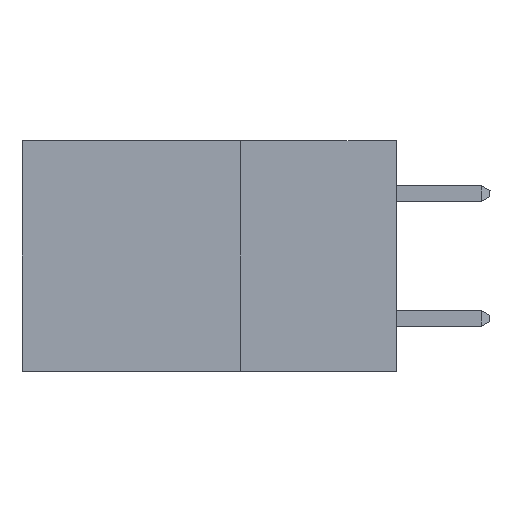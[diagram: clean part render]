
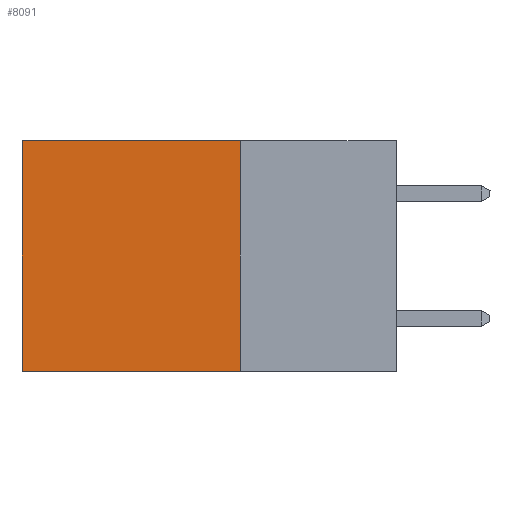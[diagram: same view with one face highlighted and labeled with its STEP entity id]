
A CAD part, left-side view. The second image highlights one B-rep face of the part: STEP entity #8091.
In plain terms, the highlighted planar face has unit normal (-1, 0, 0).
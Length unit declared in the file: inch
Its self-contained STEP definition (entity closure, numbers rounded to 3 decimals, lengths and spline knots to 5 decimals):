
#613 = CARTESIAN_POINT ( 'NONE',  ( 0.298, 0.6, 0. ) ) ;
#1604 = LINE ( 'NONE', #10227, #4846 ) ;
#1851 = DIRECTION ( 'NONE',  ( 1., 0., 0. ) ) ;
#2262 = VECTOR ( 'NONE', #8828, 39.37008 ) ;
#2681 = VECTOR ( 'NONE', #6350, 39.37008 ) ;
#2821 = VERTEX_POINT ( 'NONE', #15003 ) ;
#3408 = EDGE_LOOP ( 'NONE', ( #17617, #9028, #12761, #17676 ) ) ;
#4515 = VECTOR ( 'NONE', #17063, 39.37008 ) ;
#4846 = VECTOR ( 'NONE', #7584, 39.37008 ) ;
#4996 = CARTESIAN_POINT ( 'NONE',  ( 0.298, 0.25, -0.37 ) ) ;
#5178 = FACE_OUTER_BOUND ( 'NONE', #3408, .T. ) ;
#5921 = EDGE_CURVE ( 'NONE', #10251, #12304, #1604, .T. ) ;
#6308 = LINE ( 'NONE', #613, #2262 ) ;
#6350 = DIRECTION ( 'NONE',  ( 0., 1., 0. ) ) ;
#6814 = CARTESIAN_POINT ( 'NONE',  ( 0.298, 0.25, -0.37 ) ) ;
#7584 = DIRECTION ( 'NONE',  ( 0., 0., -1. ) ) ;
#7988 = VERTEX_POINT ( 'NONE', #8491 ) ;
#8091 = ADVANCED_FACE ( 'NONE', ( #5178 ), #16848, .F. ) ;
#8491 = CARTESIAN_POINT ( 'NONE',  ( 0.298, 0.6, 0. ) ) ;
#8533 = LINE ( 'NONE', #8878, #4515 ) ;
#8659 = CARTESIAN_POINT ( 'NONE',  ( 0.298, 0.25, 0. ) ) ;
#8828 = DIRECTION ( 'NONE',  ( 0., 0., -1. ) ) ;
#8878 = CARTESIAN_POINT ( 'NONE',  ( 0.298, 0.25, 0. ) ) ;
#9028 = ORIENTED_EDGE ( 'NONE', *, *, #12028, .F. ) ;
#9068 = CARTESIAN_POINT ( 'NONE',  ( 0.298, 0.25, 0. ) ) ;
#10227 = CARTESIAN_POINT ( 'NONE',  ( 0.298, 0.25, 0. ) ) ;
#10251 = VERTEX_POINT ( 'NONE', #9068 ) ;
#10515 = EDGE_CURVE ( 'NONE', #7988, #2821, #6308, .T. ) ;
#11417 = DIRECTION ( 'NONE',  ( 0., 0., -1. ) ) ;
#12028 = EDGE_CURVE ( 'NONE', #12304, #2821, #13603, .T. ) ;
#12304 = VERTEX_POINT ( 'NONE', #6814 ) ;
#12761 = ORIENTED_EDGE ( 'NONE', *, *, #5921, .F. ) ;
#13603 = LINE ( 'NONE', #4996, #2681 ) ;
#14401 = EDGE_CURVE ( 'NONE', #10251, #7988, #8533, .T. ) ;
#15003 = CARTESIAN_POINT ( 'NONE',  ( 0.298, 0.6, -0.37 ) ) ;
#16848 = PLANE ( 'NONE',  #16987 ) ;
#16987 = AXIS2_PLACEMENT_3D ( 'NONE', #8659, #1851, #11417 ) ;
#17063 = DIRECTION ( 'NONE',  ( 0., 1., 0. ) ) ;
#17617 = ORIENTED_EDGE ( 'NONE', *, *, #10515, .T. ) ;
#17676 = ORIENTED_EDGE ( 'NONE', *, *, #14401, .T. ) ;
